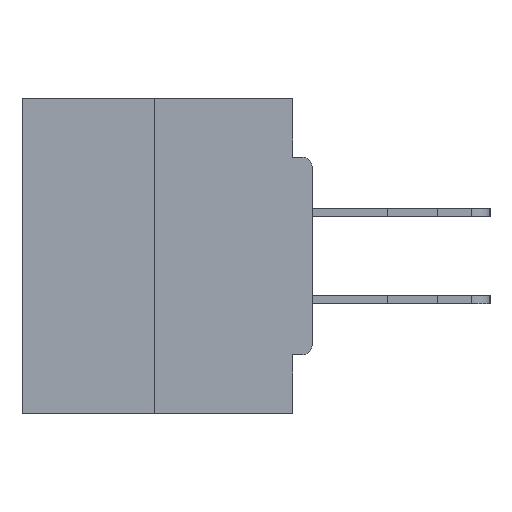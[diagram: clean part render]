
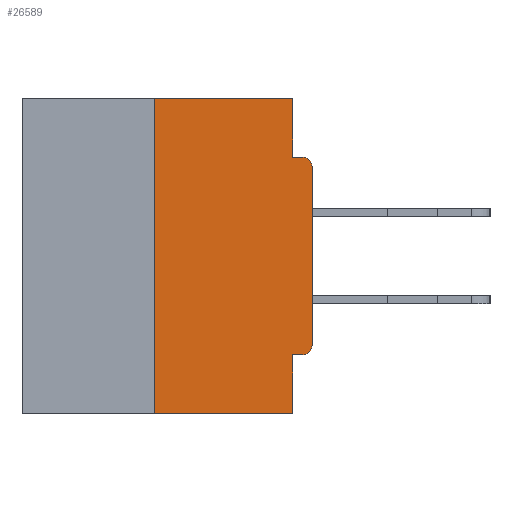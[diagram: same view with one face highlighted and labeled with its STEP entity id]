
A CAD part, left-side view. The second image highlights one B-rep face of the part: STEP entity #26589.
In plain terms, the highlighted planar face has unit normal (-1, 0, 0).
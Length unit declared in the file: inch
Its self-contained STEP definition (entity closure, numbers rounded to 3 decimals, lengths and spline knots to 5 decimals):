
#183 = CARTESIAN_POINT ( 'NONE',  ( 0., 0.46, -0.5 ) ) ;
#373 = ORIENTED_EDGE ( 'NONE', *, *, #8750, .F. ) ;
#2205 = VECTOR ( 'NONE', #3149, 39.37008 ) ;
#2765 = CARTESIAN_POINT ( 'NONE',  ( 0., 0.25, 0. ) ) ;
#2892 = CARTESIAN_POINT ( 'NONE',  ( 0., 0.015, -0.1085 ) ) ;
#2915 = CARTESIAN_POINT ( 'NONE',  ( 0., 0.46, 0. ) ) ;
#3149 = DIRECTION ( 'NONE',  ( 0., -1., 0. ) ) ;
#3386 = CARTESIAN_POINT ( 'NONE',  ( 0., 0., -0.4065 ) ) ;
#4315 = VERTEX_POINT ( 'NONE', #33994 ) ;
#4763 = CARTESIAN_POINT ( 'NONE',  ( 0., 0., -0.1085 ) ) ;
#5054 = ORIENTED_EDGE ( 'NONE', *, *, #43041, .F. ) ;
#5301 = CIRCLE ( 'NONE', #27857, 0.015 ) ;
#5526 = EDGE_CURVE ( 'NONE', #14276, #27478, #44385, .T. ) ;
#6111 = CARTESIAN_POINT ( 'NONE',  ( 0., 0., -0.0935 ) ) ;
#6266 = VERTEX_POINT ( 'NONE', #27955 ) ;
#6524 = DIRECTION ( 'NONE',  ( 0., 0., -1. ) ) ;
#6709 = VECTOR ( 'NONE', #23857, 39.37008 ) ;
#6815 = VECTOR ( 'NONE', #40726, 39.37008 ) ;
#8216 = EDGE_CURVE ( 'NONE', #14382, #11787, #12909, .T. ) ;
#8222 = VECTOR ( 'NONE', #12934, 39.37008 ) ;
#8581 = ORIENTED_EDGE ( 'NONE', *, *, #13392, .T. ) ;
#8750 = EDGE_CURVE ( 'NONE', #19546, #4315, #38344, .T. ) ;
#9148 = EDGE_CURVE ( 'NONE', #6266, #36306, #30465, .T. ) ;
#9357 = DIRECTION ( 'NONE',  ( -1., 0., 0. ) ) ;
#9586 = DIRECTION ( 'NONE',  ( 0., 0., -1. ) ) ;
#9956 = LINE ( 'NONE', #183, #6709 ) ;
#11598 = CARTESIAN_POINT ( 'NONE',  ( 0., 0.015, -0.0935 ) ) ;
#11711 = ORIENTED_EDGE ( 'NONE', *, *, #8216, .F. ) ;
#11787 = VERTEX_POINT ( 'NONE', #11598 ) ;
#12736 = CARTESIAN_POINT ( 'NONE',  ( 0., 0.25, 0. ) ) ;
#12909 = LINE ( 'NONE', #6111, #2205 ) ;
#12934 = DIRECTION ( 'NONE',  ( 0., 0., -1. ) ) ;
#13187 = CARTESIAN_POINT ( 'NONE',  ( 0., 0., 0. ) ) ;
#13392 = EDGE_CURVE ( 'NONE', #27478, #11787, #23651, .T. ) ;
#14092 = ORIENTED_EDGE ( 'NONE', *, *, #26619, .T. ) ;
#14269 = DIRECTION ( 'NONE',  ( 0., 0., -1. ) ) ;
#14276 = VERTEX_POINT ( 'NONE', #44678 ) ;
#14382 = VERTEX_POINT ( 'NONE', #35103 ) ;
#15633 = AXIS2_PLACEMENT_3D ( 'NONE', #2892, #41342, #6524 ) ;
#15682 = EDGE_CURVE ( 'NONE', #16051, #19546, #23492, .T. ) ;
#16051 = VERTEX_POINT ( 'NONE', #27074 ) ;
#16574 = CARTESIAN_POINT ( 'NONE',  ( 0., 0.031, 0. ) ) ;
#16871 = AXIS2_PLACEMENT_3D ( 'NONE', #2915, #17696, #14269 ) ;
#16875 = CARTESIAN_POINT ( 'NONE',  ( 0., 0.015, -0.3915 ) ) ;
#17696 = DIRECTION ( 'NONE',  ( 1., 0., 0. ) ) ;
#18785 = CARTESIAN_POINT ( 'NONE',  ( 0., 0.031, -0.5 ) ) ;
#19546 = VERTEX_POINT ( 'NONE', #12736 ) ;
#21270 = CARTESIAN_POINT ( 'NONE',  ( 0., 0.46, 0. ) ) ;
#22419 = LINE ( 'NONE', #18785, #34482 ) ;
#22513 = ORIENTED_EDGE ( 'NONE', *, *, #5526, .T. ) ;
#23492 = LINE ( 'NONE', #2765, #25328 ) ;
#23651 = CIRCLE ( 'NONE', #15633, 0.015 ) ;
#23857 = DIRECTION ( 'NONE',  ( 0., -1., 0. ) ) ;
#25328 = VECTOR ( 'NONE', #37121, 39.37008 ) ;
#26589 = ADVANCED_FACE ( 'NONE', ( #41362 ), #34334, .F. ) ;
#26619 = EDGE_CURVE ( 'NONE', #16051, #27876, #9956, .T. ) ;
#26828 = EDGE_LOOP ( 'NONE', ( #373, #37205, #14092, #5054, #27206, #30490, #22513, #8581, #11711, #27788 ) ) ;
#27074 = CARTESIAN_POINT ( 'NONE',  ( 0., 0.25, -0.5 ) ) ;
#27206 = ORIENTED_EDGE ( 'NONE', *, *, #9148, .F. ) ;
#27478 = VERTEX_POINT ( 'NONE', #4763 ) ;
#27788 = ORIENTED_EDGE ( 'NONE', *, *, #42357, .F. ) ;
#27857 = AXIS2_PLACEMENT_3D ( 'NONE', #16875, #9357, #9586 ) ;
#27876 = VERTEX_POINT ( 'NONE', #28358 ) ;
#27955 = CARTESIAN_POINT ( 'NONE',  ( 0., 0.015, -0.4065 ) ) ;
#28358 = CARTESIAN_POINT ( 'NONE',  ( 0., 0.031, -0.5 ) ) ;
#29020 = CARTESIAN_POINT ( 'NONE',  ( 0., 0.031, -0.4065 ) ) ;
#30465 = LINE ( 'NONE', #3386, #33998 ) ;
#30490 = ORIENTED_EDGE ( 'NONE', *, *, #31471, .T. ) ;
#31471 = EDGE_CURVE ( 'NONE', #6266, #14276, #5301, .T. ) ;
#32674 = DIRECTION ( 'NONE',  ( 0., 0., -1. ) ) ;
#33994 = CARTESIAN_POINT ( 'NONE',  ( 0., 0.031, 0. ) ) ;
#33998 = VECTOR ( 'NONE', #41363, 39.37008 ) ;
#34334 = PLANE ( 'NONE',  #16871 ) ;
#34482 = VECTOR ( 'NONE', #32674, 39.37008 ) ;
#35103 = CARTESIAN_POINT ( 'NONE',  ( 0., 0.031, -0.0935 ) ) ;
#36306 = VERTEX_POINT ( 'NONE', #29020 ) ;
#36349 = VECTOR ( 'NONE', #41767, 39.37008 ) ;
#37121 = DIRECTION ( 'NONE',  ( 0., 0., 1. ) ) ;
#37205 = ORIENTED_EDGE ( 'NONE', *, *, #15682, .F. ) ;
#38344 = LINE ( 'NONE', #21270, #36349 ) ;
#40726 = DIRECTION ( 'NONE',  ( 0., 0., 1. ) ) ;
#41342 = DIRECTION ( 'NONE',  ( -1., 0., 0. ) ) ;
#41362 = FACE_OUTER_BOUND ( 'NONE', #26828, .T. ) ;
#41363 = DIRECTION ( 'NONE',  ( 0., 1., 0. ) ) ;
#41387 = LINE ( 'NONE', #16574, #8222 ) ;
#41767 = DIRECTION ( 'NONE',  ( 0., -1., 0. ) ) ;
#42357 = EDGE_CURVE ( 'NONE', #4315, #14382, #41387, .T. ) ;
#43041 = EDGE_CURVE ( 'NONE', #36306, #27876, #22419, .T. ) ;
#44385 = LINE ( 'NONE', #13187, #6815 ) ;
#44678 = CARTESIAN_POINT ( 'NONE',  ( 0., 0., -0.3915 ) ) ;
